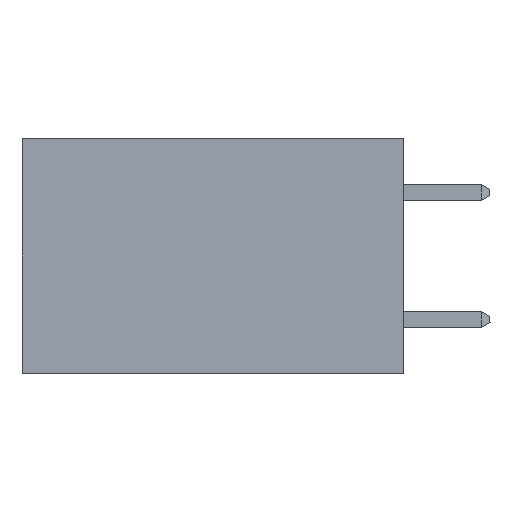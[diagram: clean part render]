
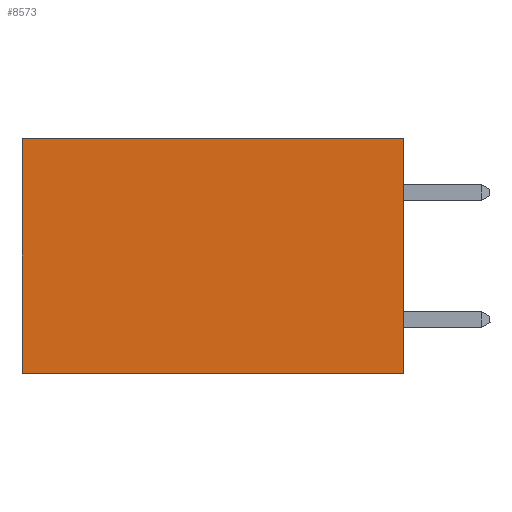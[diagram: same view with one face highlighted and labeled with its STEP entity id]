
A CAD part, left-side view. The second image highlights one B-rep face of the part: STEP entity #8573.
In plain terms, the highlighted planar face has unit normal (-1, 0, 0).
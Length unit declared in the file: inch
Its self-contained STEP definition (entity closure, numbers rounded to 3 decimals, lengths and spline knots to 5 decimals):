
#188 = CARTESIAN_POINT ( 'NONE',  ( 0.2875, 0., 0. ) ) ;
#1945 = ORIENTED_EDGE ( 'NONE', *, *, #7200, .T. ) ;
#2995 = CARTESIAN_POINT ( 'NONE',  ( 0.2875, 0.6, 0. ) ) ;
#3368 = CARTESIAN_POINT ( 'NONE',  ( 0.2875, 0., 0. ) ) ;
#4954 = CARTESIAN_POINT ( 'NONE',  ( 0.2875, 0.6, 0. ) ) ;
#6742 = CARTESIAN_POINT ( 'NONE',  ( 0.2875, 0., 0. ) ) ;
#7200 = EDGE_CURVE ( 'NONE', #17501, #13681, #43648, .T. ) ;
#8573 = ADVANCED_FACE ( 'NONE', ( #20669 ), #17311, .F. ) ;
#12264 = EDGE_CURVE ( 'NONE', #13681, #40575, #36662, .T. ) ;
#12397 = CARTESIAN_POINT ( 'NONE',  ( 0.2875, 0., 0. ) ) ;
#13681 = VERTEX_POINT ( 'NONE', #2995 ) ;
#14062 = ORIENTED_EDGE ( 'NONE', *, *, #12264, .T. ) ;
#14180 = DIRECTION ( 'NONE',  ( 1., 0., 0. ) ) ;
#15362 = DIRECTION ( 'NONE',  ( 0., 0., -1. ) ) ;
#17122 = EDGE_CURVE ( 'NONE', #29501, #40575, #39082, .T. ) ;
#17311 = PLANE ( 'NONE',  #29069 ) ;
#17501 = VERTEX_POINT ( 'NONE', #6742 ) ;
#20669 = FACE_OUTER_BOUND ( 'NONE', #32828, .T. ) ;
#22877 = VECTOR ( 'NONE', #36616, 39.37008 ) ;
#23010 = LINE ( 'NONE', #12397, #40655 ) ;
#23778 = CARTESIAN_POINT ( 'NONE',  ( 0.2875, 0.6, -0.37 ) ) ;
#24430 = CARTESIAN_POINT ( 'NONE',  ( 0.2875, 0., -0.37 ) ) ;
#24815 = DIRECTION ( 'NONE',  ( 0., 1., 0. ) ) ;
#29069 = AXIS2_PLACEMENT_3D ( 'NONE', #3368, #14180, #42283 ) ;
#29501 = VERTEX_POINT ( 'NONE', #24430 ) ;
#30096 = EDGE_CURVE ( 'NONE', #17501, #29501, #23010, .T. ) ;
#30298 = VECTOR ( 'NONE', #24815, 39.37008 ) ;
#31596 = CARTESIAN_POINT ( 'NONE',  ( 0.2875, 0., -0.37 ) ) ;
#31898 = DIRECTION ( 'NONE',  ( 0., 1., 0. ) ) ;
#32828 = EDGE_LOOP ( 'NONE', ( #14062, #35800, #35131, #1945 ) ) ;
#35131 = ORIENTED_EDGE ( 'NONE', *, *, #30096, .F. ) ;
#35800 = ORIENTED_EDGE ( 'NONE', *, *, #17122, .F. ) ;
#36616 = DIRECTION ( 'NONE',  ( 0., 0., -1. ) ) ;
#36662 = LINE ( 'NONE', #4954, #22877 ) ;
#39082 = LINE ( 'NONE', #31596, #30298 ) ;
#39803 = VECTOR ( 'NONE', #31898, 39.37008 ) ;
#40575 = VERTEX_POINT ( 'NONE', #23778 ) ;
#40655 = VECTOR ( 'NONE', #15362, 39.37008 ) ;
#42283 = DIRECTION ( 'NONE',  ( 0., 0., -1. ) ) ;
#43648 = LINE ( 'NONE', #188, #39803 ) ;
